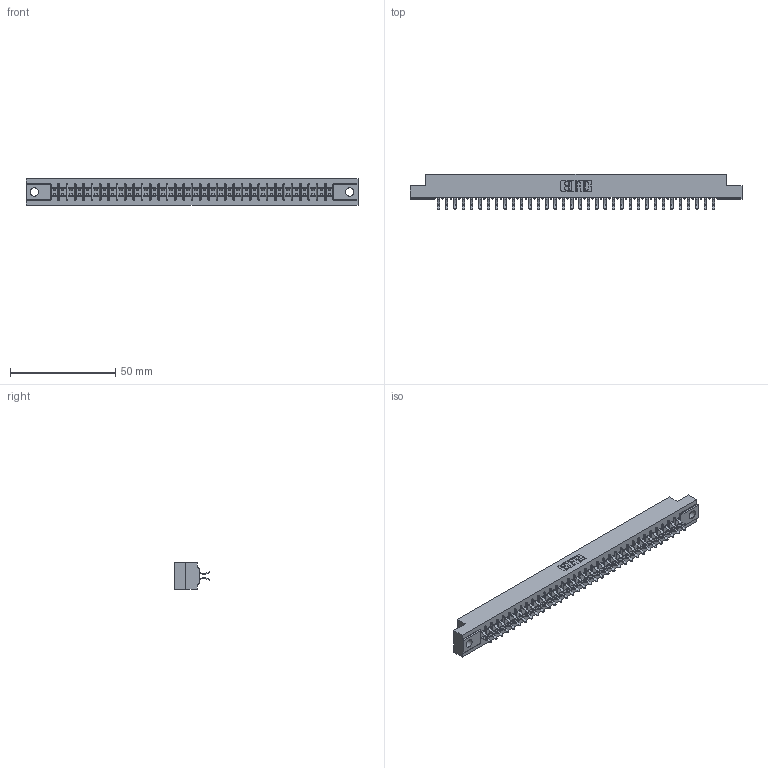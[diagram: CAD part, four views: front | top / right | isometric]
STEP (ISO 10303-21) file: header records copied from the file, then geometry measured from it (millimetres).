
FILE_DESCRIPTION (( 'STEP AP203' ), '1' );
FILE_NAME ('355-068-556-204.STEP', '2019-09-12T17:09:51', ( '' ), ( '' ), 'SwSTEP 2.0', 'SolidWorks 2016', '' );
FILE_SCHEMA (( 'CONFIG_CONTROL_DESIGN' ));
Length unit declared in the file: inch
Products named in the file (3): 305 Part_.156 Dia; 355-068-556-204; 305-290-001_556
Assembly tree (69 placements, depth 2):
  355-068-556-204
    305 Part_.156 Dia
    305-290-001_556  x68
Bounding box: 157.73 x 16.64 x 12.7 mm (x, y, z)
Volume: 16286.1 mm3; surface area: 20407.2 mm2
Topology: 69 solids, 69 shells, 3938 faces, 11334 edges, 7372 vertices
Faces by surface type: plane 2190, cylinder 1612, sphere 136
Entity records: 38427 total; most frequent: CARTESIAN_POINT 6366, ORIENTED_EDGE 6316, DIRECTION 6160, EDGE_CURVE 3158, LINE 2548, VECTOR 2548, VERTEX_POINT 2012, AXIS2_PLACEMENT_3D 1806
